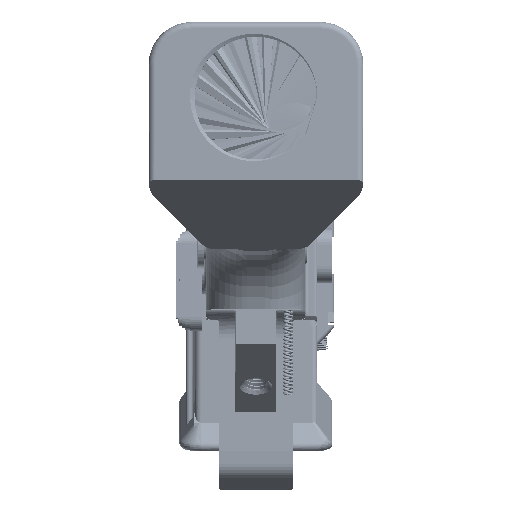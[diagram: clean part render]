
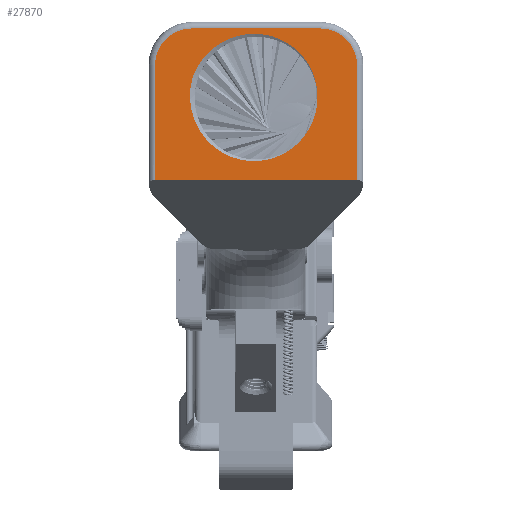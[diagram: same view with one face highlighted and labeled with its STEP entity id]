
A CAD part, front view. The second image highlights one B-rep face of the part: STEP entity #27870.
In plain terms, the highlighted planar face has unit normal (0.001, -1, 0).
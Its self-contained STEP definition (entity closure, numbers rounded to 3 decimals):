
#765=FACE_BOUND('',#4119,.T.);
#2498=FACE_OUTER_BOUND('',#4118,.T.);
#4118=EDGE_LOOP('',(#22521,#22522,#22523,#22524,#22525,#22526));
#4119=EDGE_LOOP('',(#22527,#22528,#22529));
#5581=B_SPLINE_CURVE_WITH_KNOTS('',3,(#104027,#104028,#104029,#104030,#104031,
#104032,#104033,#104034,#104035,#104036,#104037,#104038,#104039,#104040,
#104041,#104042,#104043,#104044),.UNSPECIFIED.,.F.,.F.,(4,2,2,2,2,2,2,2,
4),(0.,0.44,0.874,1.434,
1.936,2.409,2.832,3.101,3.309),
 .UNSPECIFIED.);
#5600=B_SPLINE_CURVE_WITH_KNOTS('',3,(#107705,#107706,#107707,#107708,#107709,
#107710,#107711,#107712,#107713,#107714,#107715,#107716,#107717,#107718,
#107719,#107720,#107721,#107722,#107723,#107724),.UNSPECIFIED.,.F.,.F.,
(4,2,2,2,2,2,2,2,2,4),(0.,0.38,0.774,
1.336,1.98,2.685,3.486,4.233,
4.616,5.017),.UNSPECIFIED.);
#6741=CIRCLE('',#30180,14.288);
#6867=CIRCLE('',#30467,8.5);
#6879=CIRCLE('',#30489,8.5);
#8264=LINE('',#103259,#9966);
#8268=LINE('',#106295,#9970);
#8283=LINE('',#107703,#9985);
#8284=LINE('',#107704,#9986);
#9966=VECTOR('',#35911,30.);
#9970=VECTOR('',#35937,27.295);
#9985=VECTOR('',#36044,10.);
#9986=VECTOR('',#36045,27.295);
#11890=VERTEX_POINT('',#75874);
#11891=VERTEX_POINT('',#75899);
#12384=VERTEX_POINT('',#103255);
#12385=VERTEX_POINT('',#103257);
#12387=VERTEX_POINT('',#103983);
#12397=VERTEX_POINT('',#106292);
#12398=VERTEX_POINT('',#106294);
#12418=VERTEX_POINT('',#107632);
#12431=VERTEX_POINT('',#107702);
#15359=EDGE_CURVE('',#11891,#11890,#6741,.T.);
#15981=EDGE_CURVE('',#12384,#12385,#8264,.T.);
#15983=EDGE_CURVE('',#12387,#11890,#5581,.T.);
#16000=EDGE_CURVE('',#12398,#12397,#8268,.T.);
#16010=EDGE_CURVE('',#12385,#12398,#6867,.T.);
#16035=EDGE_CURVE('',#12418,#12384,#6879,.T.);
#16054=EDGE_CURVE('',#12397,#12431,#8283,.T.);
#16055=EDGE_CURVE('',#12431,#12418,#8284,.T.);
#16056=EDGE_CURVE('',#11891,#12387,#5600,.T.);
#22521=ORIENTED_EDGE('',*,*,#16054,.T.);
#22522=ORIENTED_EDGE('',*,*,#16055,.T.);
#22523=ORIENTED_EDGE('',*,*,#16035,.T.);
#22524=ORIENTED_EDGE('',*,*,#15981,.T.);
#22525=ORIENTED_EDGE('',*,*,#16010,.T.);
#22526=ORIENTED_EDGE('',*,*,#16000,.T.);
#22527=ORIENTED_EDGE('',*,*,#15359,.T.);
#22528=ORIENTED_EDGE('',*,*,#15983,.F.);
#22529=ORIENTED_EDGE('',*,*,#16056,.F.);
#26796=PLANE('',#30506);
#27870=ADVANCED_FACE('',(#2498,#765),#26796,.T.);
#30180=AXIS2_PLACEMENT_3D('',#75900,#35129,#35130);
#30467=AXIS2_PLACEMENT_3D('',#106374,#35953,#35954);
#30489=AXIS2_PLACEMENT_3D('',#107634,#36002,#36003);
#30506=AXIS2_PLACEMENT_3D('',#107701,#36042,#36043);
#35129=DIRECTION('center_axis',(0.,1.,
0.));
#35130=DIRECTION('ref_axis',(0.,0.,-1.));
#35911=DIRECTION('',(-1.,0.,0.));
#35937=DIRECTION('',(0.,0.,-1.));
#35953=DIRECTION('center_axis',(0.,-1.,
0.));
#35954=DIRECTION('ref_axis',(0.,0.,-1.));
#36002=DIRECTION('center_axis',(0.,-1.,
0.));
#36003=DIRECTION('ref_axis',(0.,0.,-1.));
#36042=DIRECTION('center_axis',(0.,-1.,
0.));
#36043=DIRECTION('ref_axis',(0.,0.,-1.));
#36044=DIRECTION('',(1.,0.,0.));
#36045=DIRECTION('',(0.,0.,1.));
#75874=CARTESIAN_POINT('',(21.141,-81.113,18.858));
#75899=CARTESIAN_POINT('',(24.471,-81.111,28.678));
#75900=CARTESIAN_POINT('Origin',(10.198,-81.118,28.043));
#103255=CARTESIAN_POINT('',(25.195,-81.111,44.249));
#103257=CARTESIAN_POINT('',(-4.805,-81.125,44.245));
#103259=CARTESIAN_POINT('',(25.195,-81.111,44.249));
#103983=CARTESIAN_POINT('',(-4.512,-81.125,32.949));
#104027=CARTESIAN_POINT('Ctrl Pts',(-4.512,-81.125,
32.949));
#104028=CARTESIAN_POINT('Ctrl Pts',(-4.937,-81.125,
31.545));
#104029=CARTESIAN_POINT('Ctrl Pts',(-5.159,-81.125,
30.087));
#104030=CARTESIAN_POINT('Ctrl Pts',(-5.183,-81.125,
27.175));
#104031=CARTESIAN_POINT('Ctrl Pts',(-4.991,-81.125,
25.736));
#104032=CARTESIAN_POINT('Ctrl Pts',(-4.096,-81.124,
22.547));
#104033=CARTESIAN_POINT('Ctrl Pts',(-3.231,-81.124,
20.717));
#104034=CARTESIAN_POINT('Ctrl Pts',(-0.709,-81.123,
17.531));
#104035=CARTESIAN_POINT('Ctrl Pts',(0.761,-81.122,
16.268));
#104036=CARTESIAN_POINT('Ctrl Pts',(4.001,-81.121,
14.418));
#104037=CARTESIAN_POINT('Ctrl Pts',(5.871,-81.12,
13.727));
#104038=CARTESIAN_POINT('Ctrl Pts',(9.858,-81.118,
13.243));
#104039=CARTESIAN_POINT('Ctrl Pts',(11.766,-81.117,
13.381));
#104040=CARTESIAN_POINT('Ctrl Pts',(14.756,-81.116,
14.194));
#104041=CARTESIAN_POINT('Ctrl Pts',(16.281,-81.115,
14.757));
#104042=CARTESIAN_POINT('Ctrl Pts',(19.115,-81.114,
16.662));
#104043=CARTESIAN_POINT('Ctrl Pts',(20.217,-81.113,
17.684));
#104044=CARTESIAN_POINT('Ctrl Pts',(21.141,-81.113,18.858));
#106292=CARTESIAN_POINT('',(-13.299,-81.129,9.034));
#106294=CARTESIAN_POINT('',(-13.304,-81.129,35.743));
#106295=CARTESIAN_POINT('',(-13.304,-81.129,35.743));
#106374=CARTESIAN_POINT('Origin',(-4.804,-81.125,35.745));
#107632=CARTESIAN_POINT('',(33.696,-81.107,35.751));
#107634=CARTESIAN_POINT('Origin',(25.196,-81.111,35.749));
#107701=CARTESIAN_POINT('Origin',(25.196,-81.111,35.749));
#107702=CARTESIAN_POINT('',(33.701,-81.107,9.014));
#107703=CARTESIAN_POINT('',(12.602,-81.117,9.023));
#107704=CARTESIAN_POINT('',(33.701,-81.107,8.455));
#107705=CARTESIAN_POINT('Ctrl Pts',(24.471,-81.111,
28.678));
#107706=CARTESIAN_POINT('Ctrl Pts',(24.455,-81.111,
29.944));
#107707=CARTESIAN_POINT('Ctrl Pts',(24.27,-81.111,
31.203));
#107708=CARTESIAN_POINT('Ctrl Pts',(23.559,-81.112,
33.684));
#107709=CARTESIAN_POINT('Ctrl Pts',(23.022,-81.112,34.896));
#107710=CARTESIAN_POINT('Ctrl Pts',(21.359,-81.113,
37.605));
#107711=CARTESIAN_POINT('Ctrl Pts',(20.086,-81.113,
38.994));
#107712=CARTESIAN_POINT('Ctrl Pts',(16.866,-81.115,
41.381));
#107713=CARTESIAN_POINT('Ctrl Pts',(15.036,-81.116,
42.152));
#107714=CARTESIAN_POINT('Ctrl Pts',(11.449,-81.117,
43.036));
#107715=CARTESIAN_POINT('Ctrl Pts',(9.503,-81.118,
43.131));
#107716=CARTESIAN_POINT('Ctrl Pts',(5.419,-81.12,
42.536));
#107717=CARTESIAN_POINT('Ctrl Pts',(3.525,-81.121,41.772));
#107718=CARTESIAN_POINT('Ctrl Pts',(0.514,-81.122,
39.955));
#107719=CARTESIAN_POINT('Ctrl Pts',(-0.782,-81.123,
38.844));
#107720=CARTESIAN_POINT('Ctrl Pts',(-2.426,-81.124,
36.875));
#107721=CARTESIAN_POINT('Ctrl Pts',(-2.926,-81.124,
36.162));
#107722=CARTESIAN_POINT('Ctrl Pts',(-3.818,-81.124,
34.623));
#107723=CARTESIAN_POINT('Ctrl Pts',(-4.203,-81.124,
33.796));
#107724=CARTESIAN_POINT('Ctrl Pts',(-4.512,-81.125,
32.949));
